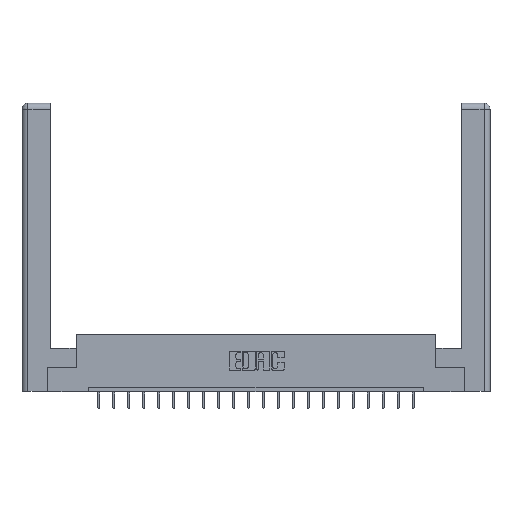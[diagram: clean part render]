
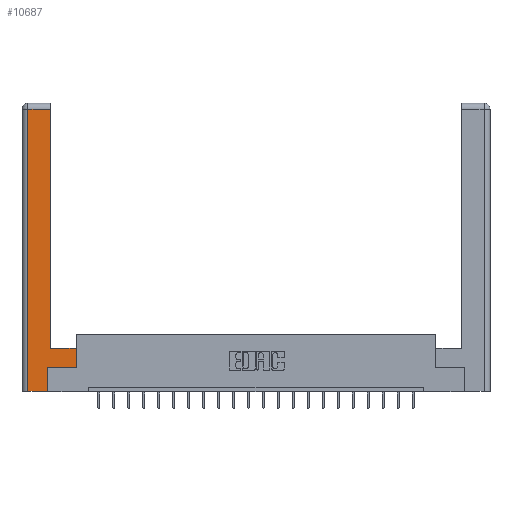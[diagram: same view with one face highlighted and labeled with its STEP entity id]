
A CAD part, top view. The second image highlights one B-rep face of the part: STEP entity #10687.
In plain terms, the highlighted planar face has unit normal (0, 0, 1).
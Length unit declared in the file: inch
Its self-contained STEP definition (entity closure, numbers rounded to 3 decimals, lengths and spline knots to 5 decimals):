
#178 = VECTOR ( 'NONE', #1392, 39.37008 ) ;
#1118 = VECTOR ( 'NONE', #5120, 39.37008 ) ;
#1392 = DIRECTION ( 'NONE',  ( 0., 1., 0. ) ) ;
#1596 = EDGE_CURVE ( 'NONE', #15826, #14945, #18198, .T. ) ;
#1849 = VERTEX_POINT ( 'NONE', #20746 ) ;
#2203 = CARTESIAN_POINT ( 'NONE',  ( 0.565, 0.245, 0. ) ) ;
#2567 = VECTOR ( 'NONE', #7168, 39.37008 ) ;
#3259 = EDGE_CURVE ( 'NONE', #5557, #19414, #21536, .T. ) ;
#3365 = CARTESIAN_POINT ( 'NONE',  ( 0.0615, 0., 0. ) ) ;
#3831 = DIRECTION ( 'NONE',  ( 1., 0., 0. ) ) ;
#3851 = DIRECTION ( 'NONE',  ( 0., 0., -1. ) ) ;
#4023 = ORIENTED_EDGE ( 'NONE', *, *, #10037, .T. ) ;
#4043 = FACE_OUTER_BOUND ( 'NONE', #13366, .T. ) ;
#4219 = CARTESIAN_POINT ( 'NONE',  ( 0.295, 0.45, 0. ) ) ;
#4290 = DIRECTION ( 'NONE',  ( -1., 0., 0. ) ) ;
#5120 = DIRECTION ( 'NONE',  ( 0., 1., 0. ) ) ;
#5288 = PLANE ( 'NONE',  #5972 ) ;
#5441 = ORIENTED_EDGE ( 'NONE', *, *, #8901, .T. ) ;
#5557 = VERTEX_POINT ( 'NONE', #15452 ) ;
#5775 = CARTESIAN_POINT ( 'NONE',  ( 0.565, 0.45, 0. ) ) ;
#5972 = AXIS2_PLACEMENT_3D ( 'NONE', #13644, #3851, #17243 ) ;
#6213 = ORIENTED_EDGE ( 'NONE', *, *, #19787, .T. ) ;
#7112 = VERTEX_POINT ( 'NONE', #13018 ) ;
#7168 = DIRECTION ( 'NONE',  ( 1., 0., 0. ) ) ;
#7337 = EDGE_CURVE ( 'NONE', #1849, #15826, #20417, .T. ) ;
#7531 = CARTESIAN_POINT ( 'NONE',  ( 0.265, 0.245, 0. ) ) ;
#7859 = CARTESIAN_POINT ( 'NONE',  ( 0.0615, 0., 0. ) ) ;
#8818 = CARTESIAN_POINT ( 'NONE',  ( 0.265, 0., 0. ) ) ;
#8901 = EDGE_CURVE ( 'NONE', #19414, #7112, #15107, .T. ) ;
#10037 = EDGE_CURVE ( 'NONE', #14945, #5557, #12709, .T. ) ;
#10687 = ADVANCED_FACE ( 'NONE', ( #4043 ), #5288, .F. ) ;
#11664 = VECTOR ( 'NONE', #15966, 39.37008 ) ;
#11731 = ORIENTED_EDGE ( 'NONE', *, *, #1596, .T. ) ;
#12379 = ORIENTED_EDGE ( 'NONE', *, *, #7337, .T. ) ;
#12709 = LINE ( 'NONE', #8818, #15311 ) ;
#12885 = ORIENTED_EDGE ( 'NONE', *, *, #17218, .T. ) ;
#13018 = CARTESIAN_POINT ( 'NONE',  ( 0.565, 0.245, 0. ) ) ;
#13320 = DIRECTION ( 'NONE',  ( -1., 0., 0. ) ) ;
#13366 = EDGE_LOOP ( 'NONE', ( #6213, #12379, #11731, #4023, #14138, #5441, #19394, #12885 ) ) ;
#13558 = EDGE_CURVE ( 'NONE', #7112, #14187, #15051, .T. ) ;
#13644 = CARTESIAN_POINT ( 'NONE',  ( 0., 0., 0. ) ) ;
#14138 = ORIENTED_EDGE ( 'NONE', *, *, #3259, .T. ) ;
#14187 = VERTEX_POINT ( 'NONE', #5775 ) ;
#14381 = VECTOR ( 'NONE', #13320, 39.37008 ) ;
#14590 = DIRECTION ( 'NONE',  ( 0., -1., 0. ) ) ;
#14945 = VERTEX_POINT ( 'NONE', #3365 ) ;
#15051 = LINE ( 'NONE', #20960, #11664 ) ;
#15107 = LINE ( 'NONE', #2203, #2567 ) ;
#15141 = CARTESIAN_POINT ( 'NONE',  ( 0.265, 0.245, 0. ) ) ;
#15311 = VECTOR ( 'NONE', #3831, 39.37008 ) ;
#15452 = CARTESIAN_POINT ( 'NONE',  ( 0.265, 0., 0. ) ) ;
#15678 = VECTOR ( 'NONE', #4290, 39.37008 ) ;
#15826 = VERTEX_POINT ( 'NONE', #16762 ) ;
#15966 = DIRECTION ( 'NONE',  ( 0., 1., 0. ) ) ;
#16357 = VECTOR ( 'NONE', #14590, 39.37008 ) ;
#16762 = CARTESIAN_POINT ( 'NONE',  ( 0.0615, 2.94, 0. ) ) ;
#17218 = EDGE_CURVE ( 'NONE', #14187, #18653, #18323, .T. ) ;
#17243 = DIRECTION ( 'NONE',  ( -1., 0., 0. ) ) ;
#17467 = CARTESIAN_POINT ( 'NONE',  ( 0.295, 3., 0. ) ) ;
#17978 = LINE ( 'NONE', #17467, #178 ) ;
#18198 = LINE ( 'NONE', #7859, #16357 ) ;
#18323 = LINE ( 'NONE', #4219, #15678 ) ;
#18527 = CARTESIAN_POINT ( 'NONE',  ( 0.0615, 2.94, 0. ) ) ;
#18653 = VERTEX_POINT ( 'NONE', #21080 ) ;
#19394 = ORIENTED_EDGE ( 'NONE', *, *, #13558, .T. ) ;
#19414 = VERTEX_POINT ( 'NONE', #7531 ) ;
#19787 = EDGE_CURVE ( 'NONE', #18653, #1849, #17978, .T. ) ;
#20417 = LINE ( 'NONE', #18527, #14381 ) ;
#20746 = CARTESIAN_POINT ( 'NONE',  ( 0.295, 2.94, 0. ) ) ;
#20960 = CARTESIAN_POINT ( 'NONE',  ( 0.565, 0.45, 0. ) ) ;
#21080 = CARTESIAN_POINT ( 'NONE',  ( 0.295, 0.45, 0. ) ) ;
#21536 = LINE ( 'NONE', #15141, #1118 ) ;
